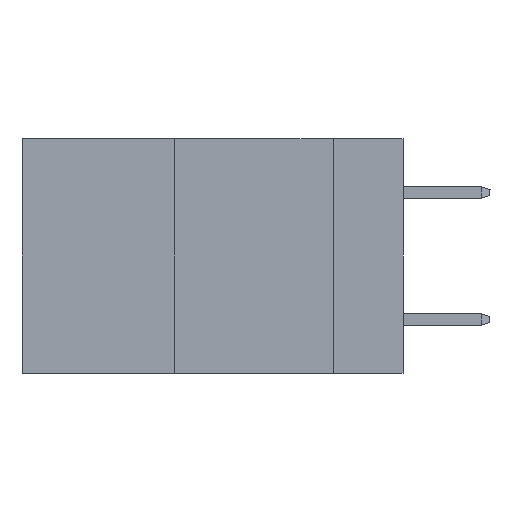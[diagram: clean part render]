
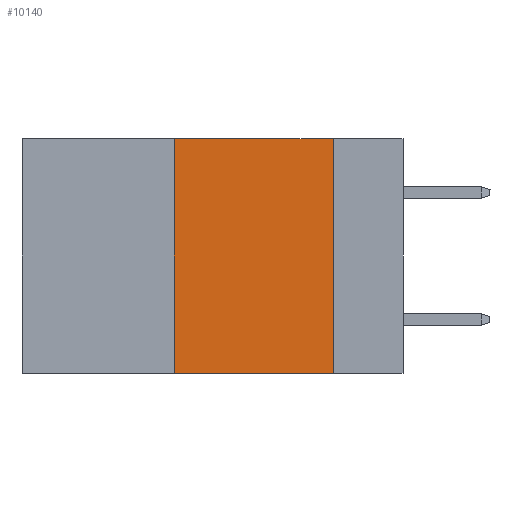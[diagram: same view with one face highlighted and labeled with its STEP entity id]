
A CAD part, left-side view. The second image highlights one B-rep face of the part: STEP entity #10140.
In plain terms, the highlighted planar face has unit normal (-1, 0, 0).
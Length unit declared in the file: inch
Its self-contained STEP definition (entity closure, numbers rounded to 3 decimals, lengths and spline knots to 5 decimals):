
#815 = ORIENTED_EDGE ( 'NONE', *, *, #14974, .F. ) ;
#882 = VECTOR ( 'NONE', #14429, 39.37008 ) ;
#1314 = CARTESIAN_POINT ( 'NONE',  ( 0., 0.36, -0.37 ) ) ;
#1437 = CARTESIAN_POINT ( 'NONE',  ( 0., 0.11, -0.37 ) ) ;
#1679 = VECTOR ( 'NONE', #7005, 39.37008 ) ;
#1799 = LINE ( 'NONE', #7649, #4216 ) ;
#2405 = LINE ( 'NONE', #14354, #1679 ) ;
#2849 = EDGE_CURVE ( 'NONE', #13467, #8223, #5642, .T. ) ;
#3179 = CARTESIAN_POINT ( 'NONE',  ( 0., 0.6, 0. ) ) ;
#4216 = VECTOR ( 'NONE', #12513, 39.37008 ) ;
#4428 = DIRECTION ( 'NONE',  ( 0., 0., -1. ) ) ;
#4745 = EDGE_CURVE ( 'NONE', #13467, #13490, #12902, .T. ) ;
#5474 = CARTESIAN_POINT ( 'NONE',  ( 0., 0.6, -0.37 ) ) ;
#5642 = LINE ( 'NONE', #5474, #16433 ) ;
#5776 = PLANE ( 'NONE',  #16371 ) ;
#6716 = VERTEX_POINT ( 'NONE', #11430 ) ;
#7005 = DIRECTION ( 'NONE',  ( 0., 0., -1. ) ) ;
#7417 = FACE_OUTER_BOUND ( 'NONE', #8953, .T. ) ;
#7649 = CARTESIAN_POINT ( 'NONE',  ( 0., 0.6, 0. ) ) ;
#8141 = ORIENTED_EDGE ( 'NONE', *, *, #12198, .F. ) ;
#8160 = ORIENTED_EDGE ( 'NONE', *, *, #2849, .T. ) ;
#8223 = VERTEX_POINT ( 'NONE', #1437 ) ;
#8953 = EDGE_LOOP ( 'NONE', ( #8141, #815, #12226, #8160 ) ) ;
#10140 = ADVANCED_FACE ( 'NONE', ( #7417 ), #5776, .F. ) ;
#11310 = DIRECTION ( 'NONE',  ( 0., -1., 0. ) ) ;
#11430 = CARTESIAN_POINT ( 'NONE',  ( 0., 0.11, 0. ) ) ;
#12198 = EDGE_CURVE ( 'NONE', #6716, #8223, #2405, .T. ) ;
#12226 = ORIENTED_EDGE ( 'NONE', *, *, #4745, .F. ) ;
#12513 = DIRECTION ( 'NONE',  ( 0., -1., 0. ) ) ;
#12902 = LINE ( 'NONE', #14237, #882 ) ;
#13423 = DIRECTION ( 'NONE',  ( 1., 0., 0. ) ) ;
#13467 = VERTEX_POINT ( 'NONE', #1314 ) ;
#13490 = VERTEX_POINT ( 'NONE', #17648 ) ;
#14237 = CARTESIAN_POINT ( 'NONE',  ( 0., 0.36, 0. ) ) ;
#14354 = CARTESIAN_POINT ( 'NONE',  ( 0., 0.11, 0. ) ) ;
#14429 = DIRECTION ( 'NONE',  ( 0., 0., 1. ) ) ;
#14974 = EDGE_CURVE ( 'NONE', #13490, #6716, #1799, .T. ) ;
#16371 = AXIS2_PLACEMENT_3D ( 'NONE', #3179, #13423, #4428 ) ;
#16433 = VECTOR ( 'NONE', #11310, 39.37008 ) ;
#17648 = CARTESIAN_POINT ( 'NONE',  ( 0., 0.36, 0. ) ) ;
